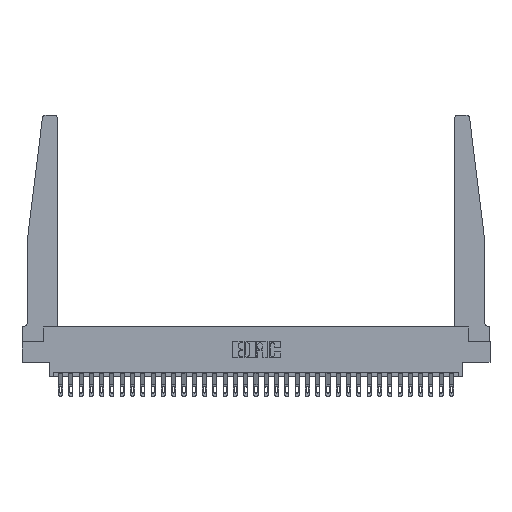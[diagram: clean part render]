
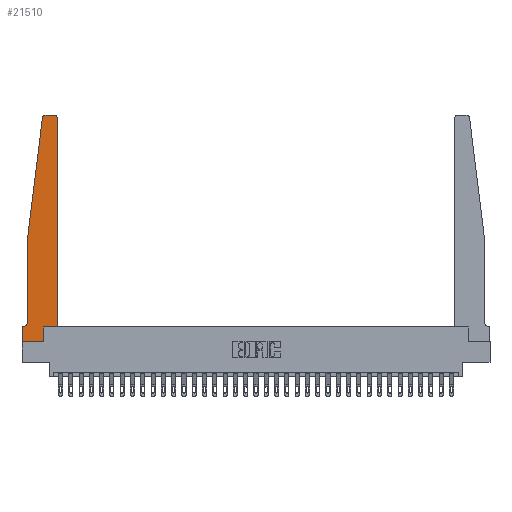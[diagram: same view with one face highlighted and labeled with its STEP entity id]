
A CAD part, top view. The second image highlights one B-rep face of the part: STEP entity #21510.
In plain terms, the highlighted planar face has unit normal (0, 0, 1).
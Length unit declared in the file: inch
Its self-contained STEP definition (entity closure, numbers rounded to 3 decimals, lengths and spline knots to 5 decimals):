
#123 = DIRECTION ( 'NONE',  ( 0., -1., 0. ) ) ;
#251 = ORIENTED_EDGE ( 'NONE', *, *, #26616, .T. ) ;
#942 = EDGE_CURVE ( 'NONE', #30565, #7117, #30013, .T. ) ;
#1378 = EDGE_CURVE ( 'NONE', #6394, #3777, #12665, .T. ) ;
#1800 = DIRECTION ( 'NONE',  ( 0., 0., -1. ) ) ;
#1871 = CARTESIAN_POINT ( 'NONE',  ( 0.395, 2.72, 0.37 ) ) ;
#2203 = CARTESIAN_POINT ( 'NONE',  ( 0., 0., 0.37 ) ) ;
#2646 = ORIENTED_EDGE ( 'NONE', *, *, #1378, .T. ) ;
#2703 = ORIENTED_EDGE ( 'NONE', *, *, #29474, .T. ) ;
#3487 = DIRECTION ( 'NONE',  ( 0., 0., 1. ) ) ;
#3495 = ORIENTED_EDGE ( 'NONE', *, *, #28081, .T. ) ;
#3777 = VERTEX_POINT ( 'NONE', #10414 ) ;
#3839 = DIRECTION ( 'NONE',  ( 1., 0., 0. ) ) ;
#3951 = ORIENTED_EDGE ( 'NONE', *, *, #24307, .T. ) ;
#4388 = EDGE_CURVE ( 'NONE', #5140, #30565, #27658, .T. ) ;
#4738 = VERTEX_POINT ( 'NONE', #20439 ) ;
#5140 = VERTEX_POINT ( 'NONE', #23879 ) ;
#5237 = EDGE_CURVE ( 'NONE', #27966, #23001, #28970, .T. ) ;
#5330 = ORIENTED_EDGE ( 'NONE', *, *, #942, .T. ) ;
#6085 = CARTESIAN_POINT ( 'NONE',  ( 0.425, 0.18, 0.37 ) ) ;
#6354 = EDGE_CURVE ( 'NONE', #7321, #5140, #13242, .T. ) ;
#6394 = VERTEX_POINT ( 'NONE', #23119 ) ;
#7096 = ORIENTED_EDGE ( 'NONE', *, *, #6354, .T. ) ;
#7117 = VERTEX_POINT ( 'NONE', #10581 ) ;
#7321 = VERTEX_POINT ( 'NONE', #8500 ) ;
#7533 = DIRECTION ( 'NONE',  ( -0.122, -0.992, 0. ) ) ;
#8099 = DIRECTION ( 'NONE',  ( 0., 0., 1. ) ) ;
#8123 = DIRECTION ( 'NONE',  ( 1., 0., 0. ) ) ;
#8317 = CARTESIAN_POINT ( 'NONE',  ( 0.065, 0.1875, 0.37 ) ) ;
#8500 = CARTESIAN_POINT ( 'NONE',  ( 0.065, 1.25, 0.37 ) ) ;
#8914 = DIRECTION ( 'NONE',  ( 0., -1., 0. ) ) ;
#9210 = DIRECTION ( 'NONE',  ( 0., 0., 1. ) ) ;
#9339 = CARTESIAN_POINT ( 'NONE',  ( 0., 0., 0.37 ) ) ;
#9379 = VECTOR ( 'NONE', #8914, 39.37008 ) ;
#9450 = LINE ( 'NONE', #19185, #28188 ) ;
#9954 = LINE ( 'NONE', #12200, #14327 ) ;
#10414 = CARTESIAN_POINT ( 'NONE',  ( 0.24675, 2.72367, 0.37 ) ) ;
#10505 = FACE_OUTER_BOUND ( 'NONE', #22760, .T. ) ;
#10581 = CARTESIAN_POINT ( 'NONE',  ( 0., 0.1875, 0.37 ) ) ;
#11375 = VERTEX_POINT ( 'NONE', #27401 ) ;
#12200 = CARTESIAN_POINT ( 'NONE',  ( 0.425, 0.18, 0.37 ) ) ;
#12665 = CIRCLE ( 'NONE', #21305, 0.03 ) ;
#12888 = PLANE ( 'NONE',  #23340 ) ;
#13242 = LINE ( 'NONE', #25528, #9379 ) ;
#14327 = VECTOR ( 'NONE', #21773, 39.37008 ) ;
#14427 = AXIS2_PLACEMENT_3D ( 'NONE', #26071, #1800, #21279 ) ;
#14902 = LINE ( 'NONE', #6085, #22155 ) ;
#15044 = ORIENTED_EDGE ( 'NONE', *, *, #4388, .T. ) ;
#15597 = CIRCLE ( 'NONE', #19676, 0.03 ) ;
#15622 = CARTESIAN_POINT ( 'NONE',  ( 0.27653, 2.72, 0.37 ) ) ;
#15994 = ORIENTED_EDGE ( 'NONE', *, *, #23464, .T. ) ;
#16567 = CARTESIAN_POINT ( 'NONE',  ( 0.2605, 0.18, 0.37 ) ) ;
#17876 = DIRECTION ( 'NONE',  ( -1., 0., 0. ) ) ;
#18407 = LINE ( 'NONE', #28149, #28462 ) ;
#18738 = DIRECTION ( 'NONE',  ( -1., 0., 0. ) ) ;
#18813 = CARTESIAN_POINT ( 'NONE',  ( 0.2605, 0., 0.37 ) ) ;
#19185 = CARTESIAN_POINT ( 'NONE',  ( 0.065, 1.25, 0.37 ) ) ;
#19286 = LINE ( 'NONE', #16567, #24848 ) ;
#19544 = DIRECTION ( 'NONE',  ( 1., 0., 0. ) ) ;
#19676 = AXIS2_PLACEMENT_3D ( 'NONE', #1871, #9210, #31074 ) ;
#19772 = LINE ( 'NONE', #2203, #24028 ) ;
#20122 = CARTESIAN_POINT ( 'NONE',  ( 0.015, 0.1875, 0.37 ) ) ;
#20224 = VERTEX_POINT ( 'NONE', #26752 ) ;
#20439 = CARTESIAN_POINT ( 'NONE',  ( 0.395, 2.75, 0.37 ) ) ;
#21180 = EDGE_CURVE ( 'NONE', #23001, #20224, #19286, .T. ) ;
#21279 = DIRECTION ( 'NONE',  ( -1., 0., 0. ) ) ;
#21305 = AXIS2_PLACEMENT_3D ( 'NONE', #15622, #3487, #8123 ) ;
#21510 = ADVANCED_FACE ( 'NONE', ( #10505 ), #12888, .T. ) ;
#21773 = DIRECTION ( 'NONE',  ( 0., 1., 0. ) ) ;
#22155 = VECTOR ( 'NONE', #3839, 39.37008 ) ;
#22173 = EDGE_CURVE ( 'NONE', #4738, #6394, #18407, .T. ) ;
#22760 = EDGE_LOOP ( 'NONE', ( #30141, #2646, #251, #7096, #15044, #5330, #3951, #26246, #30131, #3495, #15994, #2703 ) ) ;
#23001 = VERTEX_POINT ( 'NONE', #18813 ) ;
#23119 = CARTESIAN_POINT ( 'NONE',  ( 0.27653, 2.75, 0.37 ) ) ;
#23340 = AXIS2_PLACEMENT_3D ( 'NONE', #29957, #8099, #27566 ) ;
#23464 = EDGE_CURVE ( 'NONE', #11375, #25328, #9954, .T. ) ;
#23879 = CARTESIAN_POINT ( 'NONE',  ( 0.065, 0.2375, 0.37 ) ) ;
#24028 = VECTOR ( 'NONE', #123, 39.37008 ) ;
#24307 = EDGE_CURVE ( 'NONE', #7117, #27966, #19772, .T. ) ;
#24848 = VECTOR ( 'NONE', #26481, 39.37008 ) ;
#25328 = VERTEX_POINT ( 'NONE', #29388 ) ;
#25528 = CARTESIAN_POINT ( 'NONE',  ( 0.065, 1.25, 0.37 ) ) ;
#25899 = VECTOR ( 'NONE', #17876, 39.37008 ) ;
#26071 = CARTESIAN_POINT ( 'NONE',  ( 0.015, 0.2375, 0.37 ) ) ;
#26246 = ORIENTED_EDGE ( 'NONE', *, *, #5237, .T. ) ;
#26481 = DIRECTION ( 'NONE',  ( 0., 1., 0. ) ) ;
#26616 = EDGE_CURVE ( 'NONE', #3777, #7321, #9450, .T. ) ;
#26752 = CARTESIAN_POINT ( 'NONE',  ( 0.2605, 0.18, 0.37 ) ) ;
#27401 = CARTESIAN_POINT ( 'NONE',  ( 0.425, 0.18, 0.37 ) ) ;
#27566 = DIRECTION ( 'NONE',  ( 1., 0., 0. ) ) ;
#27658 = CIRCLE ( 'NONE', #14427, 0.05 ) ;
#27966 = VERTEX_POINT ( 'NONE', #29579 ) ;
#28081 = EDGE_CURVE ( 'NONE', #20224, #11375, #14902, .T. ) ;
#28149 = CARTESIAN_POINT ( 'NONE',  ( 0.25, 2.75, 0.37 ) ) ;
#28188 = VECTOR ( 'NONE', #7533, 39.37008 ) ;
#28462 = VECTOR ( 'NONE', #18738, 39.37008 ) ;
#28970 = LINE ( 'NONE', #9339, #30245 ) ;
#29388 = CARTESIAN_POINT ( 'NONE',  ( 0.425, 2.72, 0.37 ) ) ;
#29474 = EDGE_CURVE ( 'NONE', #25328, #4738, #15597, .T. ) ;
#29579 = CARTESIAN_POINT ( 'NONE',  ( 0., 0., 0.37 ) ) ;
#29957 = CARTESIAN_POINT ( 'NONE',  ( 0., 0.1875, 0.37 ) ) ;
#30013 = LINE ( 'NONE', #8317, #25899 ) ;
#30131 = ORIENTED_EDGE ( 'NONE', *, *, #21180, .T. ) ;
#30141 = ORIENTED_EDGE ( 'NONE', *, *, #22173, .T. ) ;
#30245 = VECTOR ( 'NONE', #19544, 39.37008 ) ;
#30565 = VERTEX_POINT ( 'NONE', #20122 ) ;
#31074 = DIRECTION ( 'NONE',  ( 1., 0., 0. ) ) ;
